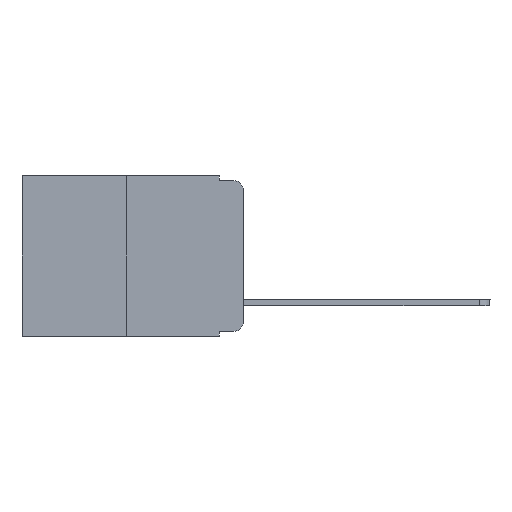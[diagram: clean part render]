
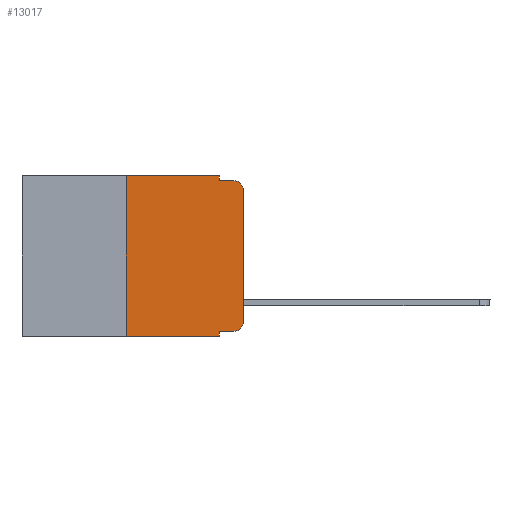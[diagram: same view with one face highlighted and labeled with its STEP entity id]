
A CAD part, left-side view. The second image highlights one B-rep face of the part: STEP entity #13017.
In plain terms, the highlighted planar face has unit normal (-1, 0, 0).
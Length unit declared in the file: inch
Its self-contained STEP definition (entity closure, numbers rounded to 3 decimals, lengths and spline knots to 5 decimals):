
#143 = CIRCLE ( 'NONE', #8977, 0.02 ) ;
#500 = CARTESIAN_POINT ( 'NONE',  ( 0., 0.051, -0.333 ) ) ;
#523 = ORIENTED_EDGE ( 'NONE', *, *, #9872, .F. ) ;
#590 = DIRECTION ( 'NONE',  ( 0., 0., -1. ) ) ;
#694 = LINE ( 'NONE', #15249, #17544 ) ;
#865 = VERTEX_POINT ( 'NONE', #9982 ) ;
#893 = DIRECTION ( 'NONE',  ( 0., -1., 0. ) ) ;
#1563 = EDGE_CURVE ( 'NONE', #10334, #11588, #2400, .T. ) ;
#1722 = DIRECTION ( 'NONE',  ( 0., -1., 0. ) ) ;
#1854 = VECTOR ( 'NONE', #3938, 39.37008 ) ;
#2027 = ORIENTED_EDGE ( 'NONE', *, *, #17132, .F. ) ;
#2127 = ORIENTED_EDGE ( 'NONE', *, *, #12574, .T. ) ;
#2219 = DIRECTION ( 'NONE',  ( 0., 0., 1. ) ) ;
#2225 = CARTESIAN_POINT ( 'NONE',  ( 0., 0., -0.313 ) ) ;
#2400 = LINE ( 'NONE', #8383, #14329 ) ;
#2644 = EDGE_CURVE ( 'NONE', #865, #6379, #694, .T. ) ;
#3140 = LINE ( 'NONE', #17510, #7613 ) ;
#3260 = ORIENTED_EDGE ( 'NONE', *, *, #7511, .T. ) ;
#3624 = VERTEX_POINT ( 'NONE', #9749 ) ;
#3739 = VECTOR ( 'NONE', #9478, 39.37008 ) ;
#3770 = LINE ( 'NONE', #4060, #12001 ) ;
#3867 = DIRECTION ( 'NONE',  ( 0., 0., -1. ) ) ;
#3905 = VECTOR ( 'NONE', #893, 39.37008 ) ;
#3938 = DIRECTION ( 'NONE',  ( 0., -1., 0. ) ) ;
#4041 = LINE ( 'NONE', #9553, #1854 ) ;
#4060 = CARTESIAN_POINT ( 'NONE',  ( 0., 0.051, 0. ) ) ;
#4127 = DIRECTION ( 'NONE',  ( -1., 0., 0. ) ) ;
#4199 = VERTEX_POINT ( 'NONE', #4491 ) ;
#4201 = EDGE_CURVE ( 'NONE', #3624, #12366, #143, .T. ) ;
#4491 = CARTESIAN_POINT ( 'NONE',  ( 0., 0.051, -0.01 ) ) ;
#4626 = EDGE_LOOP ( 'NONE', ( #3260, #5728, #523, #2027, #7305, #17734, #2127, #8898, #11773, #9657 ) ) ;
#5025 = CARTESIAN_POINT ( 'NONE',  ( 0., 0.051, -0.343 ) ) ;
#5579 = CIRCLE ( 'NONE', #8030, 0.02 ) ;
#5728 = ORIENTED_EDGE ( 'NONE', *, *, #4201, .T. ) ;
#6061 = AXIS2_PLACEMENT_3D ( 'NONE', #6844, #12960, #18662 ) ;
#6369 = CARTESIAN_POINT ( 'NONE',  ( 0., 0.051, -0.01 ) ) ;
#6379 = VERTEX_POINT ( 'NONE', #14415 ) ;
#6844 = CARTESIAN_POINT ( 'NONE',  ( 0., 0.473, 0. ) ) ;
#7305 = ORIENTED_EDGE ( 'NONE', *, *, #15856, .F. ) ;
#7376 = VECTOR ( 'NONE', #8163, 39.37008 ) ;
#7511 = EDGE_CURVE ( 'NONE', #13760, #3624, #13594, .T. ) ;
#7613 = VECTOR ( 'NONE', #1722, 39.37008 ) ;
#8030 = AXIS2_PLACEMENT_3D ( 'NONE', #14858, #13611, #590 ) ;
#8163 = DIRECTION ( 'NONE',  ( 0., 0., 1. ) ) ;
#8344 = LINE ( 'NONE', #10809, #3739 ) ;
#8383 = CARTESIAN_POINT ( 'NONE',  ( 0., 0.051, 0. ) ) ;
#8781 = CARTESIAN_POINT ( 'NONE',  ( 0., 0.02, -0.03 ) ) ;
#8898 = ORIENTED_EDGE ( 'NONE', *, *, #1563, .F. ) ;
#8977 = AXIS2_PLACEMENT_3D ( 'NONE', #8781, #4127, #10295 ) ;
#9478 = DIRECTION ( 'NONE',  ( 0., -1., 0. ) ) ;
#9553 = CARTESIAN_POINT ( 'NONE',  ( 0., 0.473, -0.343 ) ) ;
#9647 = VERTEX_POINT ( 'NONE', #17371 ) ;
#9657 = ORIENTED_EDGE ( 'NONE', *, *, #16515, .T. ) ;
#9749 = CARTESIAN_POINT ( 'NONE',  ( 0., 0., -0.03 ) ) ;
#9872 = EDGE_CURVE ( 'NONE', #4199, #12366, #10765, .T. ) ;
#9982 = CARTESIAN_POINT ( 'NONE',  ( 0., 0.25, -0.343 ) ) ;
#10153 = VERTEX_POINT ( 'NONE', #14678 ) ;
#10295 = DIRECTION ( 'NONE',  ( 0., 0., -1. ) ) ;
#10334 = VERTEX_POINT ( 'NONE', #500 ) ;
#10765 = LINE ( 'NONE', #6369, #3905 ) ;
#10809 = CARTESIAN_POINT ( 'NONE',  ( 0., 0.473, 0. ) ) ;
#11588 = VERTEX_POINT ( 'NONE', #5025 ) ;
#11773 = ORIENTED_EDGE ( 'NONE', *, *, #11863, .T. ) ;
#11863 = EDGE_CURVE ( 'NONE', #10334, #10153, #3140, .T. ) ;
#12001 = VECTOR ( 'NONE', #3867, 39.37008 ) ;
#12175 = CARTESIAN_POINT ( 'NONE',  ( 0., 0., 0. ) ) ;
#12366 = VERTEX_POINT ( 'NONE', #13571 ) ;
#12574 = EDGE_CURVE ( 'NONE', #865, #11588, #4041, .T. ) ;
#12960 = DIRECTION ( 'NONE',  ( 1., 0., 0. ) ) ;
#13017 = ADVANCED_FACE ( 'NONE', ( #15922 ), #18464, .F. ) ;
#13571 = CARTESIAN_POINT ( 'NONE',  ( 0., 0.02, -0.01 ) ) ;
#13594 = LINE ( 'NONE', #12175, #7376 ) ;
#13611 = DIRECTION ( 'NONE',  ( -1., 0., 0. ) ) ;
#13760 = VERTEX_POINT ( 'NONE', #2225 ) ;
#14092 = DIRECTION ( 'NONE',  ( 0., 0., -1. ) ) ;
#14329 = VECTOR ( 'NONE', #14092, 39.37008 ) ;
#14415 = CARTESIAN_POINT ( 'NONE',  ( 0., 0.25, 0. ) ) ;
#14678 = CARTESIAN_POINT ( 'NONE',  ( 0., 0.02, -0.333 ) ) ;
#14858 = CARTESIAN_POINT ( 'NONE',  ( 0., 0.02, -0.313 ) ) ;
#15249 = CARTESIAN_POINT ( 'NONE',  ( 0., 0.25, 0. ) ) ;
#15856 = EDGE_CURVE ( 'NONE', #6379, #9647, #8344, .T. ) ;
#15922 = FACE_OUTER_BOUND ( 'NONE', #4626, .T. ) ;
#16515 = EDGE_CURVE ( 'NONE', #10153, #13760, #5579, .T. ) ;
#17132 = EDGE_CURVE ( 'NONE', #9647, #4199, #3770, .T. ) ;
#17371 = CARTESIAN_POINT ( 'NONE',  ( 0., 0.051, 0. ) ) ;
#17510 = CARTESIAN_POINT ( 'NONE',  ( 0., 0.051, -0.333 ) ) ;
#17544 = VECTOR ( 'NONE', #2219, 39.37008 ) ;
#17734 = ORIENTED_EDGE ( 'NONE', *, *, #2644, .F. ) ;
#18464 = PLANE ( 'NONE',  #6061 ) ;
#18662 = DIRECTION ( 'NONE',  ( 0., 0., -1. ) ) ;
